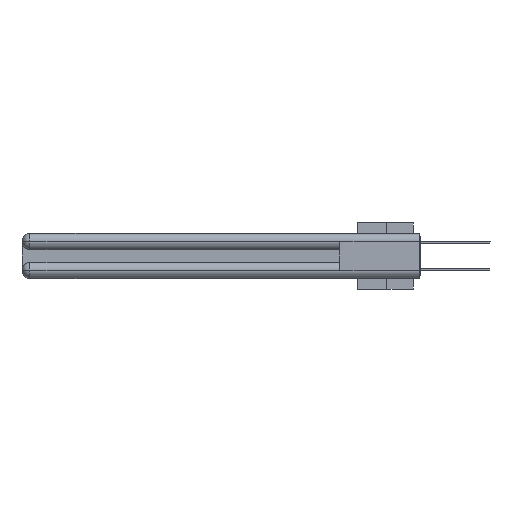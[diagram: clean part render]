
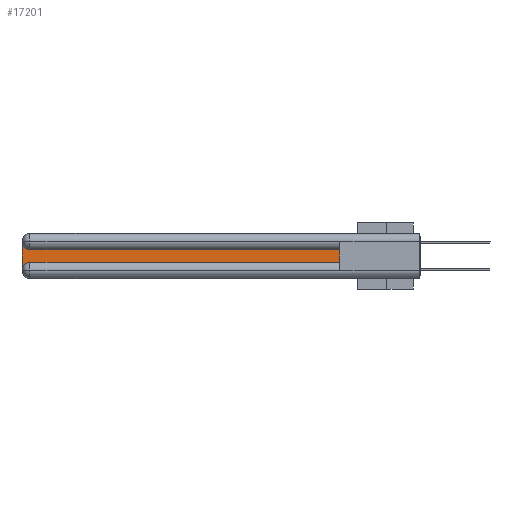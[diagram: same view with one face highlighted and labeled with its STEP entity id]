
A CAD part, left-side view. The second image highlights one B-rep face of the part: STEP entity #17201.
In plain terms, the highlighted planar face has unit normal (-1, 0, 0).
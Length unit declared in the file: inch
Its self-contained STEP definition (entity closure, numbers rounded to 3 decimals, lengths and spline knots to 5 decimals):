
#601 = VERTEX_POINT ( 'NONE', #5688 ) ;
#1063 = VECTOR ( 'NONE', #25756, 39.37008 ) ;
#1712 = LINE ( 'NONE', #12848, #24779 ) ;
#3787 = PLANE ( 'NONE',  #25189 ) ;
#4080 = VECTOR ( 'NONE', #34602, 39.37008 ) ;
#5688 = CARTESIAN_POINT ( 'NONE',  ( 0.075, 3., -0.0625 ) ) ;
#6153 = CARTESIAN_POINT ( 'NONE',  ( 0.075, 2.94, -0.0625 ) ) ;
#6386 = AXIS2_PLACEMENT_3D ( 'NONE', #32807, #21433, #16516 ) ;
#6623 = LINE ( 'NONE', #31138, #4080 ) ;
#8288 = VERTEX_POINT ( 'NONE', #33314 ) ;
#8755 = EDGE_CURVE ( 'NONE', #8288, #26173, #10963, .T. ) ;
#8759 = CARTESIAN_POINT ( 'NONE',  ( 0.075, 0.6, -0.1225 ) ) ;
#8908 = CIRCLE ( 'NONE', #14753, 0.06 ) ;
#10307 = EDGE_CURVE ( 'NONE', #27982, #12718, #32151, .T. ) ;
#10963 = LINE ( 'NONE', #8759, #13822 ) ;
#11822 = DIRECTION ( 'NONE',  ( 0., 0., -1. ) ) ;
#12003 = DIRECTION ( 'NONE',  ( 1., 0., 0. ) ) ;
#12718 = VERTEX_POINT ( 'NONE', #32241 ) ;
#12848 = CARTESIAN_POINT ( 'NONE',  ( 0.075, 3., -0.2175 ) ) ;
#13822 = VECTOR ( 'NONE', #22270, 39.37008 ) ;
#14603 = CARTESIAN_POINT ( 'NONE',  ( 0.075, 0.6, -0.2175 ) ) ;
#14750 = DIRECTION ( 'NONE',  ( 1., 0., 0. ) ) ;
#14753 = AXIS2_PLACEMENT_3D ( 'NONE', #6153, #14750, #33960 ) ;
#16516 = DIRECTION ( 'NONE',  ( 0., 0., -1. ) ) ;
#17201 = ADVANCED_FACE ( 'NONE', ( #20205 ), #3787, .F. ) ;
#18606 = EDGE_CURVE ( 'NONE', #26173, #601, #8908, .T. ) ;
#19375 = ORIENTED_EDGE ( 'NONE', *, *, #10307, .T. ) ;
#19610 = ORIENTED_EDGE ( 'NONE', *, *, #23169, .T. ) ;
#19661 = ORIENTED_EDGE ( 'NONE', *, *, #8755, .T. ) ;
#20019 = ORIENTED_EDGE ( 'NONE', *, *, #24753, .T. ) ;
#20205 = FACE_OUTER_BOUND ( 'NONE', #30634, .T. ) ;
#21433 = DIRECTION ( 'NONE',  ( 1., 0., 0. ) ) ;
#21874 = VERTEX_POINT ( 'NONE', #31492 ) ;
#21891 = CARTESIAN_POINT ( 'NONE',  ( 0.075, 2.94, -0.1225 ) ) ;
#21985 = ORIENTED_EDGE ( 'NONE', *, *, #18606, .T. ) ;
#22129 = CIRCLE ( 'NONE', #6386, 0.06 ) ;
#22270 = DIRECTION ( 'NONE',  ( 0., 1., 0. ) ) ;
#22397 = CARTESIAN_POINT ( 'NONE',  ( 0.075, 2.94, -0.2175 ) ) ;
#23049 = ORIENTED_EDGE ( 'NONE', *, *, #30992, .T. ) ;
#23169 = EDGE_CURVE ( 'NONE', #12718, #8288, #6623, .T. ) ;
#23987 = DIRECTION ( 'NONE',  ( 0., 0., -1. ) ) ;
#24753 = EDGE_CURVE ( 'NONE', #21874, #27982, #22129, .T. ) ;
#24779 = VECTOR ( 'NONE', #23987, 39.37008 ) ;
#25189 = AXIS2_PLACEMENT_3D ( 'NONE', #33762, #12003, #11822 ) ;
#25756 = DIRECTION ( 'NONE',  ( 0., -1., 0. ) ) ;
#26173 = VERTEX_POINT ( 'NONE', #21891 ) ;
#27982 = VERTEX_POINT ( 'NONE', #22397 ) ;
#30634 = EDGE_LOOP ( 'NONE', ( #19661, #21985, #23049, #20019, #19375, #19610 ) ) ;
#30992 = EDGE_CURVE ( 'NONE', #601, #21874, #1712, .T. ) ;
#31138 = CARTESIAN_POINT ( 'NONE',  ( 0.075, 0.6, -0.2175 ) ) ;
#31492 = CARTESIAN_POINT ( 'NONE',  ( 0.075, 3., -0.2775 ) ) ;
#32151 = LINE ( 'NONE', #14603, #1063 ) ;
#32241 = CARTESIAN_POINT ( 'NONE',  ( 0.075, 0.6, -0.2175 ) ) ;
#32807 = CARTESIAN_POINT ( 'NONE',  ( 0.075, 2.94, -0.2775 ) ) ;
#33314 = CARTESIAN_POINT ( 'NONE',  ( 0.075, 0.6, -0.1225 ) ) ;
#33762 = CARTESIAN_POINT ( 'NONE',  ( 0.075, 3., -0.1225 ) ) ;
#33960 = DIRECTION ( 'NONE',  ( 0., 0., -1. ) ) ;
#34602 = DIRECTION ( 'NONE',  ( 0., 0., 1. ) ) ;
